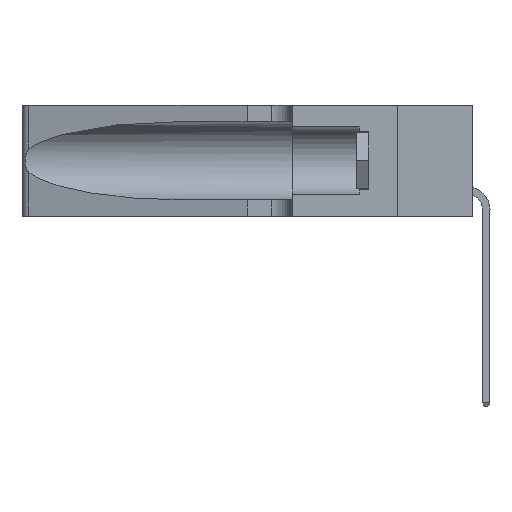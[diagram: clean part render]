
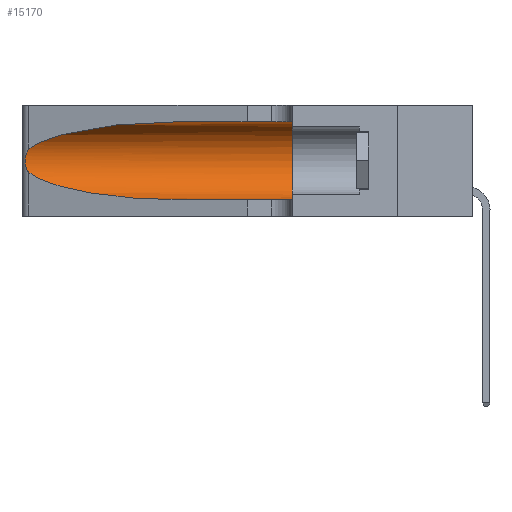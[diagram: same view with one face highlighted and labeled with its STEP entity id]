
A CAD part, left-side view. The second image highlights one B-rep face of the part: STEP entity #15170.
In plain terms, the highlighted cylindrical face has radius 3.308 mm (diameter 6.617 mm), a partial arc.
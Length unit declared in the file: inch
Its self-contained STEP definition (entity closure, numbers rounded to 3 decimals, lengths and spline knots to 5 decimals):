
#97 = ORIENTED_EDGE ( 'NONE', *, *, #32044, .F. ) ;
#126 = CARTESIAN_POINT ( 'NONE',  ( 0.1305, 0.35, 0.31525 ) ) ;
#277 = CYLINDRICAL_SURFACE ( 'NONE', #556, 0.13025 ) ;
#279 = LINE ( 'NONE', #19762, #24158 ) ;
#556 = AXIS2_PLACEMENT_3D ( 'NONE', #31360, #22578, #37809 ) ;
#1798 = VERTEX_POINT ( 'NONE', #29414 ) ;
#2630 = VERTEX_POINT ( 'NONE', #9371 ) ;
#3556 = CARTESIAN_POINT ( 'NONE',  ( 0.1305, 0.35, 0.185 ) ) ;
#3996 = CARTESIAN_POINT ( 'NONE',  ( 0.25555, 1.22993, 0.14849 ) ) ;
#4796 = CARTESIAN_POINT ( 'NONE',  ( 0.26018, 1.23835, 0.19895 ) ) ;
#4814 = B_SPLINE_CURVE_WITH_KNOTS ( 'NONE', 3,
 ( #36426, #12373, #36067, #12260, #12636, #4796, #27695, #27525, #27926, #22063, #37416, #19068, #3996, #10317 ),
 .UNSPECIFIED., .F., .F.,
 ( 4, 2, 2, 2, 2, 2, 4 ),
 ( 0., 0.00027, 0.00053, 0.00107, 0.0016, 0.00187, 0.00214 ),
 .UNSPECIFIED. ) ;
#5803 = ORIENTED_EDGE ( 'NONE', *, *, #9439, .T. ) ;
#6852 = DIRECTION ( 'NONE',  ( 0., 0., 1. ) ) ;
#7888 = CARTESIAN_POINT ( 'NONE',  ( 0.1305, 0.72297, 0.31525 ) ) ;
#9371 = CARTESIAN_POINT ( 'NONE',  ( 0.1305, 0.72297, 0.05475 ) ) ;
#9439 = EDGE_CURVE ( 'NONE', #2630, #20525, #9578, .T. ) ;
#9578 = LINE ( 'NONE', #12958, #23624 ) ;
#9858 = DIRECTION ( 'NONE',  ( 0., 1., 0. ) ) ;
#10062 = DIRECTION ( 'NONE',  ( 0., -1., 0. ) ) ;
#10317 = CARTESIAN_POINT ( 'NONE',  ( 0.25487, 1.22718, 0.14631 ) ) ;
#11137 = EDGE_CURVE ( 'NONE', #1798, #16547, #4814, .T. ) ;
#11594 = AXIS2_PLACEMENT_3D ( 'NONE', #3556, #9858, #6852 ) ;
#12260 = CARTESIAN_POINT ( 'NONE',  ( 0.25787, 1.23484, 0.2124 ) ) ;
#12373 = CARTESIAN_POINT ( 'NONE',  ( 0.25555, 1.22994, 0.2215 ) ) ;
#12507 = CARTESIAN_POINT ( 'NONE',  ( 0.18966, 0.96281, 0.05475 ) ) ;
#12636 = CARTESIAN_POINT ( 'NONE',  ( 0.25854, 1.2359, 0.20912 ) ) ;
#12958 = CARTESIAN_POINT ( 'NONE',  ( 0.1305, 1.61858, 0.05475 ) ) ;
#15170 = ADVANCED_FACE ( 'NONE', ( #22322 ), #277, .F. ) ;
#15904 = EDGE_CURVE ( 'NONE', #16547, #2630, #29067, .T. ) ;
#16547 = VERTEX_POINT ( 'NONE', #36002 ) ;
#16554 = ORIENTED_EDGE ( 'NONE', *, *, #17172, .T. ) ;
#16926 = CARTESIAN_POINT ( 'NONE',  ( 0.18966, 0.96281, 0.31525 ) ) ;
#17172 = EDGE_CURVE ( 'NONE', #27031, #1798, #18693, .T. ) ;
#17364 = ORIENTED_EDGE ( 'NONE', *, *, #26871, .F. ) ;
#18146 = CIRCLE ( 'NONE', #11594, 0.13025 ) ;
#18693 =( BOUNDED_CURVE ( )  B_SPLINE_CURVE ( 3, ( #7888, #16926, #26037, #29074 ),
 .UNSPECIFIED., .F., .T. ) 
 B_SPLINE_CURVE_WITH_KNOTS ( ( 4, 4 ),
 ( 1.5708, 2.84003 ),
 .UNSPECIFIED. ) 
 CURVE ( )  GEOMETRIC_REPRESENTATION_ITEM ( )  RATIONAL_B_SPLINE_CURVE ( ( 1., 0.87, 0.87, 1. ) ) 
 REPRESENTATION_ITEM ( '' )  );
#19068 = CARTESIAN_POINT ( 'NONE',  ( 0.25639, 1.23186, 0.15144 ) ) ;
#19762 = CARTESIAN_POINT ( 'NONE',  ( 0.1305, 1.61858, 0.31525 ) ) ;
#20525 = VERTEX_POINT ( 'NONE', #33723 ) ;
#22063 = CARTESIAN_POINT ( 'NONE',  ( 0.25856, 1.23593, 0.16098 ) ) ;
#22322 = FACE_OUTER_BOUND ( 'NONE', #30897, .T. ) ;
#22578 = DIRECTION ( 'NONE',  ( 0., -1., 0. ) ) ;
#23624 = VECTOR ( 'NONE', #10062, 39.37008 ) ;
#23994 = CARTESIAN_POINT ( 'NONE',  ( 0.25487, 1.22718, 0.14631 ) ) ;
#24158 = VECTOR ( 'NONE', #35079, 39.37008 ) ;
#25098 = ORIENTED_EDGE ( 'NONE', *, *, #11137, .T. ) ;
#26037 = CARTESIAN_POINT ( 'NONE',  ( 0.2373, 1.15595, 0.28018 ) ) ;
#26634 = CARTESIAN_POINT ( 'NONE',  ( 0.1305, 0.72297, 0.31525 ) ) ;
#26871 = EDGE_CURVE ( 'NONE', #27031, #35792, #279, .T. ) ;
#27031 = VERTEX_POINT ( 'NONE', #26634 ) ;
#27525 = CARTESIAN_POINT ( 'NONE',  ( 0.26075, 1.23896, 0.178 ) ) ;
#27695 = CARTESIAN_POINT ( 'NONE',  ( 0.26075, 1.23896, 0.19203 ) ) ;
#27926 = CARTESIAN_POINT ( 'NONE',  ( 0.26017, 1.23833, 0.17102 ) ) ;
#29067 =( BOUNDED_CURVE ( )  B_SPLINE_CURVE ( 3, ( #23994, #33294, #12507, #36072 ),
 .UNSPECIFIED., .F., .T. ) 
 B_SPLINE_CURVE_WITH_KNOTS ( ( 4, 4 ),
 ( 3.44316, 4.71239 ),
 .UNSPECIFIED. ) 
 CURVE ( )  GEOMETRIC_REPRESENTATION_ITEM ( )  RATIONAL_B_SPLINE_CURVE ( ( 1., 0.87, 0.87, 1. ) ) 
 REPRESENTATION_ITEM ( '' )  );
#29074 = CARTESIAN_POINT ( 'NONE',  ( 0.25487, 1.22718, 0.22369 ) ) ;
#29414 = CARTESIAN_POINT ( 'NONE',  ( 0.25487, 1.22718, 0.22369 ) ) ;
#30897 = EDGE_LOOP ( 'NONE', ( #16554, #25098, #37052, #5803, #97, #17364 ) ) ;
#31360 = CARTESIAN_POINT ( 'NONE',  ( 0.1305, 1.61858, 0.185 ) ) ;
#32044 = EDGE_CURVE ( 'NONE', #35792, #20525, #18146, .T. ) ;
#33294 = CARTESIAN_POINT ( 'NONE',  ( 0.2373, 1.15595, 0.08982 ) ) ;
#33723 = CARTESIAN_POINT ( 'NONE',  ( 0.1305, 0.35, 0.05475 ) ) ;
#35079 = DIRECTION ( 'NONE',  ( 0., -1., 0. ) ) ;
#35792 = VERTEX_POINT ( 'NONE', #126 ) ;
#36002 = CARTESIAN_POINT ( 'NONE',  ( 0.25487, 1.22718, 0.14631 ) ) ;
#36067 = CARTESIAN_POINT ( 'NONE',  ( 0.25639, 1.23184, 0.21858 ) ) ;
#36072 = CARTESIAN_POINT ( 'NONE',  ( 0.1305, 0.72297, 0.05475 ) ) ;
#36426 = CARTESIAN_POINT ( 'NONE',  ( 0.25487, 1.22718, 0.22369 ) ) ;
#37052 = ORIENTED_EDGE ( 'NONE', *, *, #15904, .T. ) ;
#37416 = CARTESIAN_POINT ( 'NONE',  ( 0.25789, 1.23486, 0.15765 ) ) ;
#37809 = DIRECTION ( 'NONE',  ( 0., 0., -1. ) ) ;
